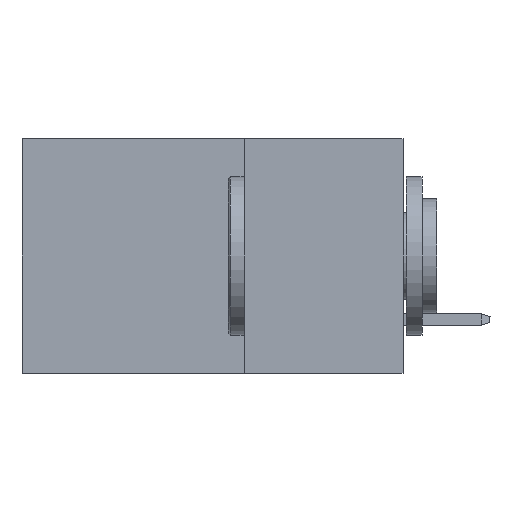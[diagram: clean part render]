
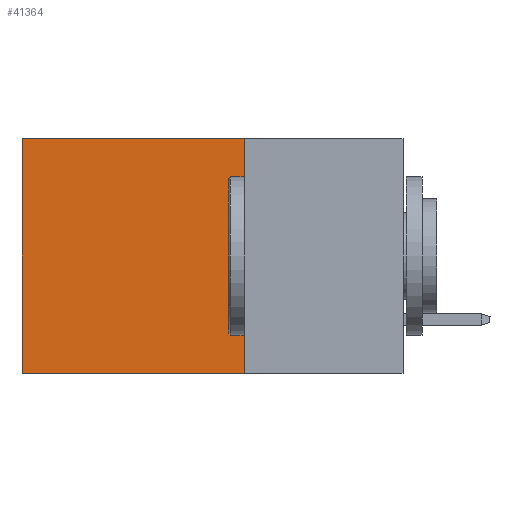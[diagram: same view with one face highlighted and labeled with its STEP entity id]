
A CAD part, left-side view. The second image highlights one B-rep face of the part: STEP entity #41364.
In plain terms, the highlighted planar face has unit normal (-1, 0, 0).
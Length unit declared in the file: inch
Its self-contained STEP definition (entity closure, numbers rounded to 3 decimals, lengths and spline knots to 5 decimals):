
#691 = EDGE_LOOP ( 'NONE', ( #44823, #30019, #45380, #32619 ) ) ;
#2193 = EDGE_CURVE ( 'NONE', #5724, #43039, #48761, .T. ) ;
#2404 = DIRECTION ( 'NONE',  ( 0., 0., -1. ) ) ;
#2865 = VERTEX_POINT ( 'NONE', #16825 ) ;
#2970 = CARTESIAN_POINT ( 'NONE',  ( 0.2875, 0.25, 0. ) ) ;
#5724 = VERTEX_POINT ( 'NONE', #23774 ) ;
#7332 = DIRECTION ( 'NONE',  ( 0., 0., -1. ) ) ;
#11159 = LINE ( 'NONE', #14985, #42933 ) ;
#14985 = CARTESIAN_POINT ( 'NONE',  ( 0.2875, 0.25, -0.37 ) ) ;
#16825 = CARTESIAN_POINT ( 'NONE',  ( 0.2875, 0.6, -0.37 ) ) ;
#18326 = CARTESIAN_POINT ( 'NONE',  ( 0.2875, 0.25, 0. ) ) ;
#19283 = DIRECTION ( 'NONE',  ( 0., 1., 0. ) ) ;
#19775 = EDGE_CURVE ( 'NONE', #43039, #2865, #11159, .T. ) ;
#21981 = FACE_OUTER_BOUND ( 'NONE', #691, .T. ) ;
#23774 = CARTESIAN_POINT ( 'NONE',  ( 0.2875, 0.25, 0. ) ) ;
#24826 = VECTOR ( 'NONE', #33017, 39.37008 ) ;
#26006 = VERTEX_POINT ( 'NONE', #26296 ) ;
#26296 = CARTESIAN_POINT ( 'NONE',  ( 0.2875, 0.6, 0. ) ) ;
#30019 = ORIENTED_EDGE ( 'NONE', *, *, #19775, .F. ) ;
#32619 = ORIENTED_EDGE ( 'NONE', *, *, #41749, .T. ) ;
#33017 = DIRECTION ( 'NONE',  ( 0., 0., -1. ) ) ;
#35767 = AXIS2_PLACEMENT_3D ( 'NONE', #2970, #50061, #7332 ) ;
#35802 = VECTOR ( 'NONE', #19283, 39.37008 ) ;
#36751 = VECTOR ( 'NONE', #2404, 39.37008 ) ;
#38402 = DIRECTION ( 'NONE',  ( 0., 1., 0. ) ) ;
#38812 = CARTESIAN_POINT ( 'NONE',  ( 0.2875, 0.25, 0. ) ) ;
#41364 = ADVANCED_FACE ( 'NONE', ( #21981 ), #45714, .F. ) ;
#41749 = EDGE_CURVE ( 'NONE', #5724, #26006, #42488, .T. ) ;
#42488 = LINE ( 'NONE', #38812, #35802 ) ;
#42933 = VECTOR ( 'NONE', #38402, 39.37008 ) ;
#43039 = VERTEX_POINT ( 'NONE', #50409 ) ;
#44823 = ORIENTED_EDGE ( 'NONE', *, *, #49718, .T. ) ;
#44931 = CARTESIAN_POINT ( 'NONE',  ( 0.2875, 0.6, 0. ) ) ;
#45380 = ORIENTED_EDGE ( 'NONE', *, *, #2193, .F. ) ;
#45692 = LINE ( 'NONE', #44931, #24826 ) ;
#45714 = PLANE ( 'NONE',  #35767 ) ;
#48761 = LINE ( 'NONE', #18326, #36751 ) ;
#49718 = EDGE_CURVE ( 'NONE', #26006, #2865, #45692, .T. ) ;
#50061 = DIRECTION ( 'NONE',  ( 1., 0., 0. ) ) ;
#50409 = CARTESIAN_POINT ( 'NONE',  ( 0.2875, 0.25, -0.37 ) ) ;
